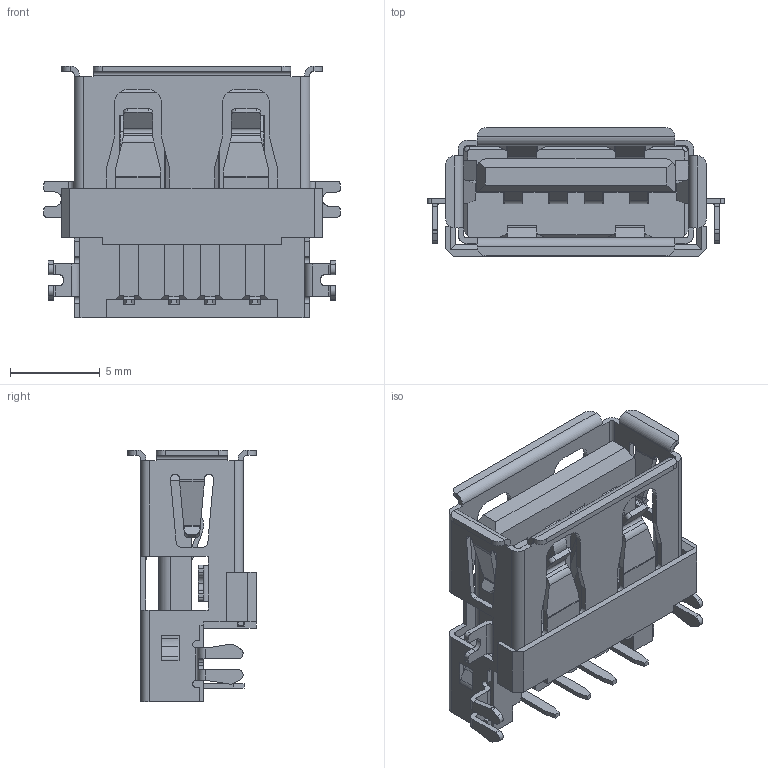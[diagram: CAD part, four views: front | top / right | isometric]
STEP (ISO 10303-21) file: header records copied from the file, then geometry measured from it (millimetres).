
FILE_DESCRIPTION (( 'STEP AP214' ), '1' );
FILE_NAME ('690G104-159-041.STEP', '2021-01-14T13:25:20', ( '' ), ( '' ), 'SwSTEP 2.0', 'SolidWorks 2020', '' );
FILE_SCHEMA (( 'AUTOMOTIVE_DESIGN' ));
Length unit declared in the file: millimetre
Products named in the file (4): Shell 690G104-X59-04X; 690G104-159-041; Insulator 690G104-X59-04X_Black; Contacts 690G104-X59-04X
Assembly tree (3 placements, depth 2):
  690G104-159-041
    Insulator 690G104-X59-04X_Black
    Contacts 690G104-X59-04X
    Shell 690G104-X59-04X
Bounding box: 16.5 x 7.12 x 14 mm (x, y, z)
Volume: 424.1 mm3; surface area: 1770.9 mm2
Topology: 6 solids, 6 shells, 831 faces, 2381 edges, 1547 vertices
Faces by surface type: plane 604, cylinder 201, bspline 24, cone 2
Entity records: 28225 total; most frequent: CARTESIAN_POINT 6528, ORIENTED_EDGE 4762, DIRECTION 4094, EDGE_CURVE 2381, LINE 1892, VECTOR 1892, VERTEX_POINT 1547, AXIS2_PLACEMENT_3D 1101
